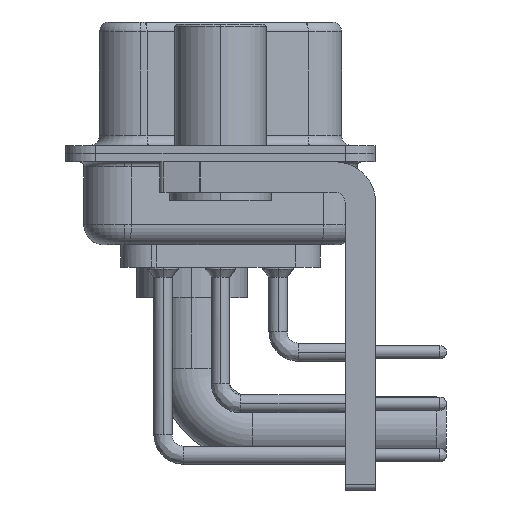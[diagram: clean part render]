
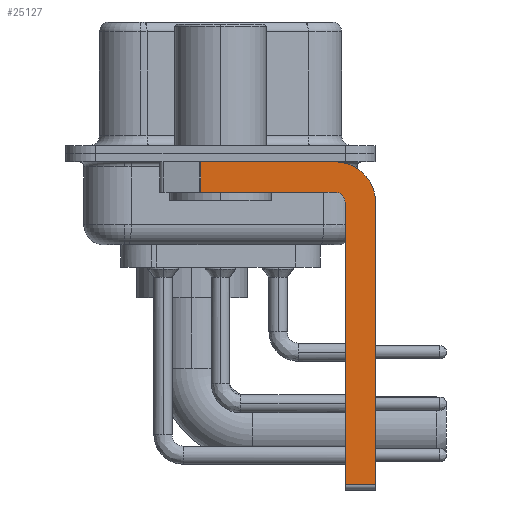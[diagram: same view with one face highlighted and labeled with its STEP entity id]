
A CAD part, left-side view. The second image highlights one B-rep face of the part: STEP entity #25127.
In plain terms, the highlighted planar face has unit normal (-1, 0, 0).
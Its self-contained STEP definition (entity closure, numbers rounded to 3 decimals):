
#401 = DIRECTION ( 'NONE',  ( 0., 0., -1. ) ) ;
#505 = ORIENTED_EDGE ( 'NONE', *, *, #30776, .F. ) ;
#658 = CARTESIAN_POINT ( 'NONE',  ( -2.9, 0.978, -1.9 ) ) ;
#2269 = CARTESIAN_POINT ( 'NONE',  ( -2.9, 3., -0.4 ) ) ;
#2775 = VERTEX_POINT ( 'NONE', #4921 ) ;
#3430 = CARTESIAN_POINT ( 'NONE',  ( -2.9, -5.65, -1.9 ) ) ;
#3462 = CARTESIAN_POINT ( 'NONE',  ( -2.9, -5.65, -16.35 ) ) ;
#3506 = VERTEX_POINT ( 'NONE', #3430 ) ;
#4490 = DIRECTION ( 'NONE',  ( -1., 0., 0. ) ) ;
#4921 = CARTESIAN_POINT ( 'NONE',  ( -2.9, -7.65, -16.35 ) ) ;
#5013 = CARTESIAN_POINT ( 'NONE',  ( -2.9, -5.65, -1.9 ) ) ;
#5825 = CARTESIAN_POINT ( 'NONE',  ( -2.9, -6.15, -16.35 ) ) ;
#5998 = ORIENTED_EDGE ( 'NONE', *, *, #17168, .F. ) ;
#6151 = VERTEX_POINT ( 'NONE', #5825 ) ;
#6199 = EDGE_CURVE ( 'NONE', #6151, #2775, #27402, .T. ) ;
#7242 = DIRECTION ( 'NONE',  ( 0., 0., 1. ) ) ;
#8380 = DIRECTION ( 'NONE',  ( 0., 0., -1. ) ) ;
#8451 = VECTOR ( 'NONE', #31515, 1000. ) ;
#10083 = ORIENTED_EDGE ( 'NONE', *, *, #17061, .F. ) ;
#10392 = VERTEX_POINT ( 'NONE', #34639 ) ;
#12420 = EDGE_CURVE ( 'NONE', #37548, #15621, #31896, .T. ) ;
#12537 = CARTESIAN_POINT ( 'NONE',  ( -2.9, -7.65, -2.4 ) ) ;
#14236 = DIRECTION ( 'NONE',  ( 0., 1., 0. ) ) ;
#14862 = FACE_OUTER_BOUND ( 'NONE', #32144, .T. ) ;
#15009 = DIRECTION ( 'NONE',  ( 1., 0., 0. ) ) ;
#15621 = VERTEX_POINT ( 'NONE', #17396 ) ;
#15700 = CARTESIAN_POINT ( 'NONE',  ( -2.9, -5.65, -2.4 ) ) ;
#16978 = ORIENTED_EDGE ( 'NONE', *, *, #22926, .T. ) ;
#17061 = EDGE_CURVE ( 'NONE', #15621, #2775, #30581, .T. ) ;
#17168 = EDGE_CURVE ( 'NONE', #32868, #3506, #33302, .T. ) ;
#17396 = CARTESIAN_POINT ( 'NONE',  ( -2.9, -7.65, -2.4 ) ) ;
#17611 = CARTESIAN_POINT ( 'NONE',  ( -2.9, -5.65, -2.4 ) ) ;
#18193 = PLANE ( 'NONE',  #26192 ) ;
#18721 = ORIENTED_EDGE ( 'NONE', *, *, #20522, .F. ) ;
#20522 = EDGE_CURVE ( 'NONE', #10392, #37548, #38338, .T. ) ;
#21443 = CARTESIAN_POINT ( 'NONE',  ( -2.9, -6.15, -2.4 ) ) ;
#22243 = ORIENTED_EDGE ( 'NONE', *, *, #12420, .F. ) ;
#22926 = EDGE_CURVE ( 'NONE', #10392, #37097, #27288, .T. ) ;
#24728 = VECTOR ( 'NONE', #24861, 1000. ) ;
#24861 = DIRECTION ( 'NONE',  ( 0., -1., 0. ) ) ;
#25127 = ADVANCED_FACE ( 'NONE', ( #14862 ), #18193, .F. ) ;
#26192 = AXIS2_PLACEMENT_3D ( 'NONE', #17611, #35427, #8380 ) ;
#26250 = CARTESIAN_POINT ( 'NONE',  ( -2.9, -6.15, -16.6 ) ) ;
#27288 = LINE ( 'NONE', #27673, #32394 ) ;
#27373 = ORIENTED_EDGE ( 'NONE', *, *, #6199, .T. ) ;
#27402 = LINE ( 'NONE', #3462, #24728 ) ;
#27673 = CARTESIAN_POINT ( 'NONE',  ( -2.9, 0.978, -1.9 ) ) ;
#30198 = DIRECTION ( 'NONE',  ( 0., 0., -1. ) ) ;
#30581 = LINE ( 'NONE', #12537, #36469 ) ;
#30776 = EDGE_CURVE ( 'NONE', #6151, #32868, #34500, .T. ) ;
#30852 = EDGE_CURVE ( 'NONE', #3506, #37097, #35206, .T. ) ;
#31296 = AXIS2_PLACEMENT_3D ( 'NONE', #36158, #15009, #33044 ) ;
#31515 = DIRECTION ( 'NONE',  ( 0., -1., 0. ) ) ;
#31896 = CIRCLE ( 'NONE', #31296, 2. ) ;
#32144 = EDGE_LOOP ( 'NONE', ( #18721, #16978, #33954, #5998, #505, #27373, #10083, #22243 ) ) ;
#32394 = VECTOR ( 'NONE', #401, 1000. ) ;
#32590 = CARTESIAN_POINT ( 'NONE',  ( -2.9, -5.65, -0.4 ) ) ;
#32868 = VERTEX_POINT ( 'NONE', #21443 ) ;
#33044 = DIRECTION ( 'NONE',  ( 0., 0., -1. ) ) ;
#33302 = CIRCLE ( 'NONE', #38286, 0.5 ) ;
#33954 = ORIENTED_EDGE ( 'NONE', *, *, #30852, .F. ) ;
#34500 = LINE ( 'NONE', #26250, #35955 ) ;
#34639 = CARTESIAN_POINT ( 'NONE',  ( -2.9, 0.978, -0.4 ) ) ;
#35206 = LINE ( 'NONE', #5013, #36629 ) ;
#35427 = DIRECTION ( 'NONE',  ( 1., 0., 0. ) ) ;
#35955 = VECTOR ( 'NONE', #37613, 1000. ) ;
#36158 = CARTESIAN_POINT ( 'NONE',  ( -2.9, -5.65, -2.4 ) ) ;
#36469 = VECTOR ( 'NONE', #30198, 1000. ) ;
#36629 = VECTOR ( 'NONE', #14236, 1000. ) ;
#37097 = VERTEX_POINT ( 'NONE', #658 ) ;
#37548 = VERTEX_POINT ( 'NONE', #32590 ) ;
#37613 = DIRECTION ( 'NONE',  ( 0., 0., 1. ) ) ;
#38286 = AXIS2_PLACEMENT_3D ( 'NONE', #15700, #4490, #7242 ) ;
#38338 = LINE ( 'NONE', #2269, #8451 ) ;
